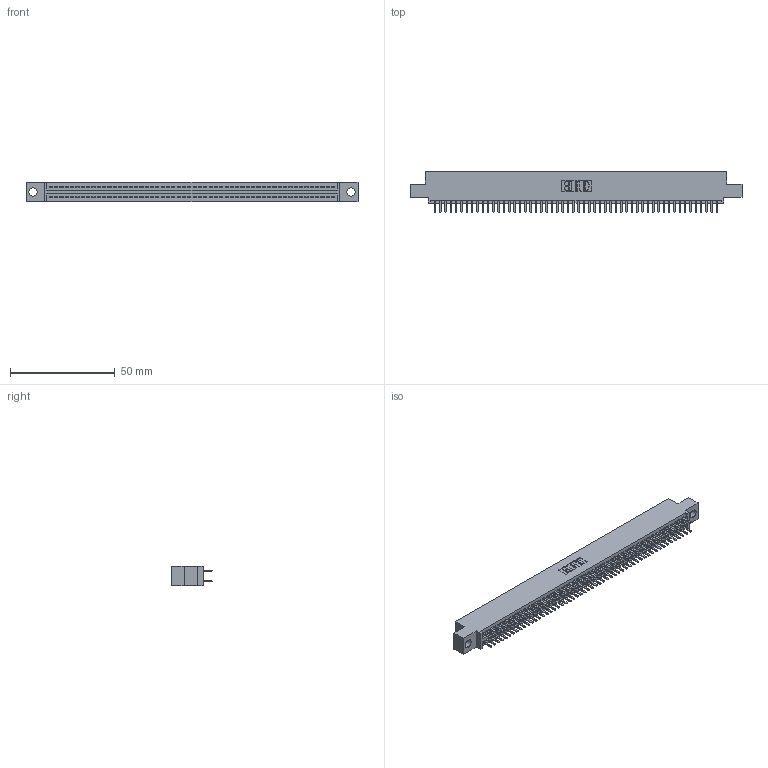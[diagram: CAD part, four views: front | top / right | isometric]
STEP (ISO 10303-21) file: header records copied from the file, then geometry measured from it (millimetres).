
FILE_DESCRIPTION (( 'STEP AP203' ), '1' );
FILE_NAME ('395-108-520-504.STEP', '2021-06-17T16:55:53', ( '' ), ( '' ), 'SwSTEP 2.0', 'SolidWorks 2020', '' );
FILE_SCHEMA (( 'CONFIG_CONTROL_DESIGN' ));
Length unit declared in the file: inch
Products named in the file (3): 345-292-001_345-293-120; 395-108-520-504; 345 Part_0.110 Offset - 0.156 Dia-TI
Assembly tree (109 placements, depth 2):
  395-108-520-504
    345 Part_0.110 Offset - 0.156 Dia-TI
    345-292-001_345-293-120  x108
Bounding box: 158.37 x 19.68 x 9.4 mm (x, y, z)
Volume: 15268.7 mm3; surface area: 22645.6 mm2
Topology: 109 solids, 109 shells, 5976 faces, 17345 edges, 11274 vertices
Faces by surface type: plane 3878, cylinder 2098
Entity records: 41419 total; most frequent: CARTESIAN_POINT 6950, ORIENTED_EDGE 6870, DIRECTION 6099, EDGE_CURVE 3435, VECTOR 3083, LINE 3083, VERTEX_POINT 2286, AXIS2_PLACEMENT_3D 1508
